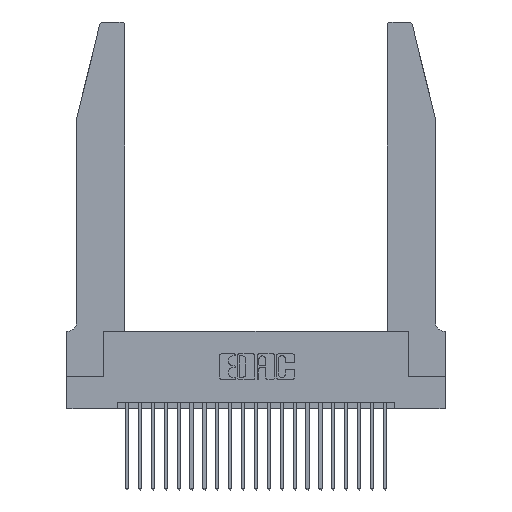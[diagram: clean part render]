
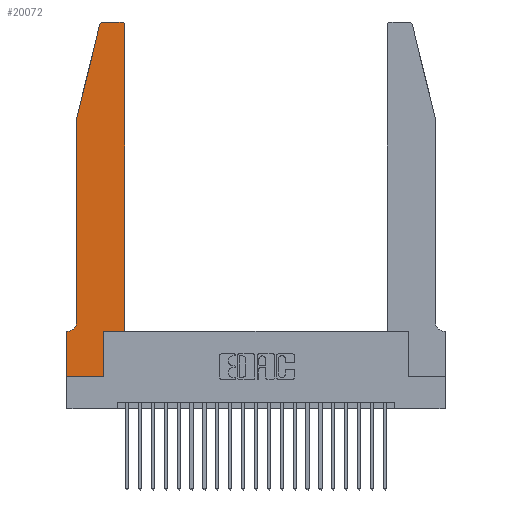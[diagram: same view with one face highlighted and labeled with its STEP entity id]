
A CAD part, top view. The second image highlights one B-rep face of the part: STEP entity #20072.
In plain terms, the highlighted planar face has unit normal (0, 0, 1).
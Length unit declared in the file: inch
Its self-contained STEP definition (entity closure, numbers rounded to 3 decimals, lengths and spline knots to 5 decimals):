
#200 = ORIENTED_EDGE ( 'NONE', *, *, #18376, .T. ) ;
#204 = VECTOR ( 'NONE', #5028, 39.37008 ) ;
#644 = VECTOR ( 'NONE', #8440, 39.37008 ) ;
#1158 = ORIENTED_EDGE ( 'NONE', *, *, #21033, .T. ) ;
#1268 = CARTESIAN_POINT ( 'NONE',  ( 0.0755, 2., 0.37 ) ) ;
#1425 = DIRECTION ( 'NONE',  ( 0., 0., 1. ) ) ;
#1757 = VECTOR ( 'NONE', #9454, 39.37008 ) ;
#1871 = DIRECTION ( 'NONE',  ( 1., 0., 0. ) ) ;
#1951 = VECTOR ( 'NONE', #7606, 39.37008 ) ;
#2060 = LINE ( 'NONE', #4948, #11397 ) ;
#2104 = VERTEX_POINT ( 'NONE', #23496 ) ;
#2172 = CARTESIAN_POINT ( 'NONE',  ( 0., 0., 0.37 ) ) ;
#2379 = FACE_OUTER_BOUND ( 'NONE', #8607, .T. ) ;
#2723 = ORIENTED_EDGE ( 'NONE', *, *, #4272, .T. ) ;
#2783 = CARTESIAN_POINT ( 'NONE',  ( 0.0755, 0.42, 0.37 ) ) ;
#2984 = EDGE_CURVE ( 'NONE', #22311, #2104, #20949, .T. ) ;
#3076 = ORIENTED_EDGE ( 'NONE', *, *, #6272, .T. ) ;
#3610 = CARTESIAN_POINT ( 'NONE',  ( 0.0755, 0.35, 0.37 ) ) ;
#4272 = EDGE_CURVE ( 'NONE', #8430, #12165, #16612, .T. ) ;
#4553 = EDGE_CURVE ( 'NONE', #23032, #19335, #10197, .T. ) ;
#4861 = EDGE_CURVE ( 'NONE', #12165, #12061, #8152, .T. ) ;
#4888 = CARTESIAN_POINT ( 'NONE',  ( 0.2865, 0.35, 0.37 ) ) ;
#4948 = CARTESIAN_POINT ( 'NONE',  ( 0.4505, 0.35, 0.37 ) ) ;
#4999 = CARTESIAN_POINT ( 'NONE',  ( 0.4205, 2.75, 0.37 ) ) ;
#5028 = DIRECTION ( 'NONE',  ( 0., -1., 0. ) ) ;
#5134 = LINE ( 'NONE', #21375, #644 ) ;
#5289 = LINE ( 'NONE', #1268, #204 ) ;
#6176 = VECTOR ( 'NONE', #12860, 39.37008 ) ;
#6196 = CARTESIAN_POINT ( 'NONE',  ( 0.0055, 0.42, 0.37 ) ) ;
#6272 = EDGE_CURVE ( 'NONE', #24028, #23032, #6908, .T. ) ;
#6778 = DIRECTION ( 'NONE',  ( 1., 0., 0. ) ) ;
#6908 = LINE ( 'NONE', #14984, #1951 ) ;
#7423 = ORIENTED_EDGE ( 'NONE', *, *, #21025, .T. ) ;
#7487 = ORIENTED_EDGE ( 'NONE', *, *, #12727, .T. ) ;
#7511 = CARTESIAN_POINT ( 'NONE',  ( 0.0055, 0.35, 0.37 ) ) ;
#7606 = DIRECTION ( 'NONE',  ( -1., 0., 0. ) ) ;
#7673 = EDGE_CURVE ( 'NONE', #19335, #22637, #12710, .T. ) ;
#8080 = DIRECTION ( 'NONE',  ( -1., 0., 0. ) ) ;
#8152 = LINE ( 'NONE', #23396, #13106 ) ;
#8430 = VERTEX_POINT ( 'NONE', #2172 ) ;
#8433 = LINE ( 'NONE', #19137, #12805 ) ;
#8440 = DIRECTION ( 'NONE',  ( 0., 1., 0. ) ) ;
#8601 = CARTESIAN_POINT ( 'NONE',  ( 0.2865, 0., 0.37 ) ) ;
#8607 = EDGE_LOOP ( 'NONE', ( #3076, #15372, #22367, #15974, #200, #11534, #1158, #2723, #21144, #7487, #14261, #7423 ) ) ;
#8637 = CARTESIAN_POINT ( 'NONE',  ( 0.0755, 2., 0.37 ) ) ;
#8672 = CARTESIAN_POINT ( 'NONE',  ( 0.25487, 2.72718, 0.37 ) ) ;
#9420 = CIRCLE ( 'NONE', #11478, 0.07 ) ;
#9454 = DIRECTION ( 'NONE',  ( 1., 0., 0. ) ) ;
#9907 = CARTESIAN_POINT ( 'NONE',  ( 0.4205, 2.72, 0.37 ) ) ;
#10197 = CIRCLE ( 'NONE', #19490, 0.03 ) ;
#10513 = DIRECTION ( 'NONE',  ( 0., 1., 0. ) ) ;
#10524 = DIRECTION ( 'NONE',  ( -0.239, -0.971, 0. ) ) ;
#11301 = CARTESIAN_POINT ( 'NONE',  ( 0.284, 2.75, 0.37 ) ) ;
#11397 = VECTOR ( 'NONE', #6778, 39.37008 ) ;
#11478 = AXIS2_PLACEMENT_3D ( 'NONE', #6196, #19175, #8080 ) ;
#11534 = ORIENTED_EDGE ( 'NONE', *, *, #2984, .T. ) ;
#11784 = DIRECTION ( 'NONE',  ( 1., 0., 0. ) ) ;
#12061 = VERTEX_POINT ( 'NONE', #4888 ) ;
#12127 = CARTESIAN_POINT ( 'NONE',  ( 0.0755, 2., 0.37 ) ) ;
#12165 = VERTEX_POINT ( 'NONE', #8601 ) ;
#12631 = CARTESIAN_POINT ( 'NONE',  ( 0., 0.35, 0.37 ) ) ;
#12710 = LINE ( 'NONE', #8637, #17058 ) ;
#12727 = EDGE_CURVE ( 'NONE', #12061, #20345, #2060, .T. ) ;
#12796 = EDGE_CURVE ( 'NONE', #22637, #16789, #5289, .T. ) ;
#12805 = VECTOR ( 'NONE', #20976, 39.37008 ) ;
#12860 = DIRECTION ( 'NONE',  ( -1., 0., 0. ) ) ;
#13041 = DIRECTION ( 'NONE',  ( 0., 0., 1. ) ) ;
#13106 = VECTOR ( 'NONE', #10513, 39.37008 ) ;
#13967 = CIRCLE ( 'NONE', #21405, 0.03 ) ;
#14261 = ORIENTED_EDGE ( 'NONE', *, *, #17298, .T. ) ;
#14498 = DIRECTION ( 'NONE',  ( 1., 0., 0. ) ) ;
#14984 = CARTESIAN_POINT ( 'NONE',  ( 0.2605, 2.75, 0.37 ) ) ;
#15372 = ORIENTED_EDGE ( 'NONE', *, *, #4553, .T. ) ;
#15974 = ORIENTED_EDGE ( 'NONE', *, *, #12796, .T. ) ;
#16612 = LINE ( 'NONE', #20562, #1757 ) ;
#16789 = VERTEX_POINT ( 'NONE', #2783 ) ;
#16849 = VERTEX_POINT ( 'NONE', #21477 ) ;
#17058 = VECTOR ( 'NONE', #10524, 39.37008 ) ;
#17298 = EDGE_CURVE ( 'NONE', #20345, #16849, #5134, .T. ) ;
#18376 = EDGE_CURVE ( 'NONE', #16789, #22311, #9420, .T. ) ;
#18907 = CARTESIAN_POINT ( 'NONE',  ( 0.4505, 0.35, 0.37 ) ) ;
#19091 = AXIS2_PLACEMENT_3D ( 'NONE', #12631, #1425, #14498 ) ;
#19137 = CARTESIAN_POINT ( 'NONE',  ( 0., 0., 0.37 ) ) ;
#19175 = DIRECTION ( 'NONE',  ( 0., 0., -1. ) ) ;
#19335 = VERTEX_POINT ( 'NONE', #8672 ) ;
#19490 = AXIS2_PLACEMENT_3D ( 'NONE', #24051, #13041, #1871 ) ;
#20072 = ADVANCED_FACE ( 'NONE', ( #2379 ), #23630, .T. ) ;
#20345 = VERTEX_POINT ( 'NONE', #18907 ) ;
#20562 = CARTESIAN_POINT ( 'NONE',  ( 0., 0., 0.37 ) ) ;
#20949 = LINE ( 'NONE', #3610, #6176 ) ;
#20976 = DIRECTION ( 'NONE',  ( 0., -1., 0. ) ) ;
#21025 = EDGE_CURVE ( 'NONE', #16849, #24028, #13967, .T. ) ;
#21033 = EDGE_CURVE ( 'NONE', #2104, #8430, #8433, .T. ) ;
#21144 = ORIENTED_EDGE ( 'NONE', *, *, #4861, .T. ) ;
#21375 = CARTESIAN_POINT ( 'NONE',  ( 0.4505, 0.35, 0.37 ) ) ;
#21405 = AXIS2_PLACEMENT_3D ( 'NONE', #9907, #22800, #11784 ) ;
#21477 = CARTESIAN_POINT ( 'NONE',  ( 0.4505, 2.72, 0.37 ) ) ;
#22311 = VERTEX_POINT ( 'NONE', #7511 ) ;
#22367 = ORIENTED_EDGE ( 'NONE', *, *, #7673, .T. ) ;
#22637 = VERTEX_POINT ( 'NONE', #12127 ) ;
#22800 = DIRECTION ( 'NONE',  ( 0., 0., 1. ) ) ;
#23032 = VERTEX_POINT ( 'NONE', #11301 ) ;
#23396 = CARTESIAN_POINT ( 'NONE',  ( 0.2865, 0.35, 0.37 ) ) ;
#23496 = CARTESIAN_POINT ( 'NONE',  ( 0., 0.35, 0.37 ) ) ;
#23630 = PLANE ( 'NONE',  #19091 ) ;
#24028 = VERTEX_POINT ( 'NONE', #4999 ) ;
#24051 = CARTESIAN_POINT ( 'NONE',  ( 0.284, 2.72, 0.37 ) ) ;
